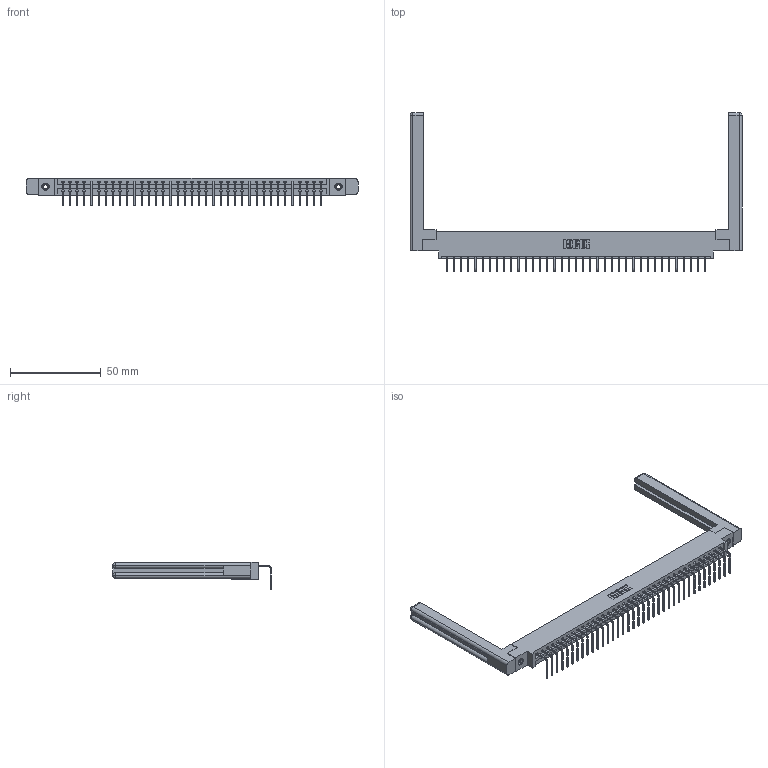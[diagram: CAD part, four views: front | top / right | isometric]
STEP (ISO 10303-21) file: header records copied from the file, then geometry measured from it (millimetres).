
FILE_DESCRIPTION (( 'STEP AP203' ), '1' );
FILE_NAME ('337-037-558-658.STEP', '2019-10-07T14:42:38', ( '' ), ( '' ), 'SwSTEP 2.0', 'SolidWorks 2016', '' );
FILE_SCHEMA (( 'CONFIG_CONTROL_DESIGN' ));
Length unit declared in the file: inch
Products named in the file (5): 345-292-001_558 Tail - 2; 345-250-001_345-250-001-102; 307-220-058; 337-037-558-658; 337 Part_0.170 Offset - 0.156 Dia-TI
Assembly tree (42 placements, depth 2):
  337-037-558-658
    337 Part_0.170 Offset - 0.156 Dia-TI
    345-292-001_558 Tail - 2  x37
    345-250-001_345-250-001-102  x2
    307-220-058  x2
Bounding box: 183.24 x 87.57 x 15.37 mm (x, y, z)
Volume: 26149.6 mm3; surface area: 25659.8 mm2
Topology: 42 solids, 42 shells, 2628 faces, 7855 edges, 5174 vertices
Faces by surface type: plane 1934, cylinder 670, cone 12, torus 12
Entity records: 31000 total; most frequent: CARTESIAN_POINT 5400, ORIENTED_EDGE 5312, DIRECTION 4574, EDGE_CURVE 2656, LINE 2480, VECTOR 2480, VERTEX_POINT 1762, AXIS2_PLACEMENT_3D 1047
